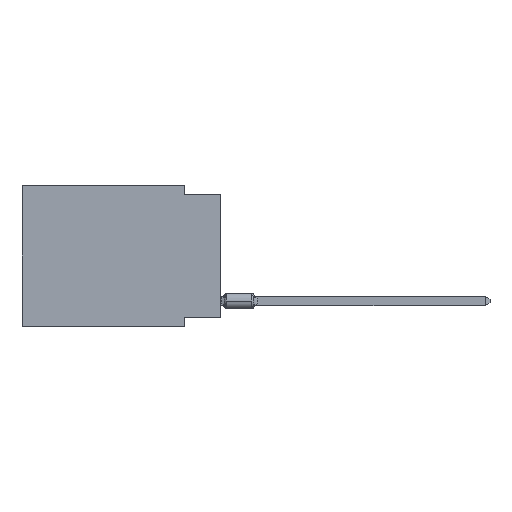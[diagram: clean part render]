
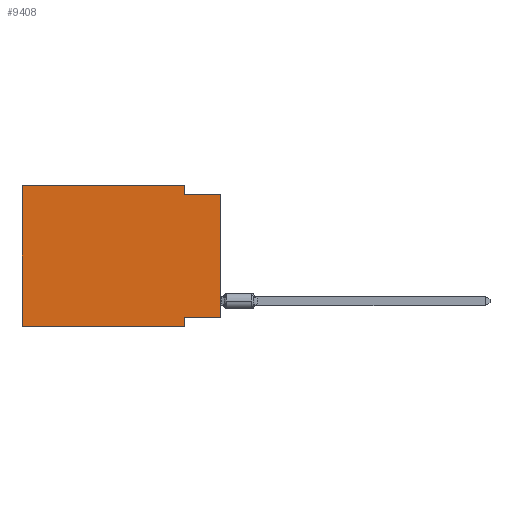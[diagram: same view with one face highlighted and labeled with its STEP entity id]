
A CAD part, left-side view. The second image highlights one B-rep face of the part: STEP entity #9408.
In plain terms, the highlighted planar face has unit normal (-1, 0, 0).
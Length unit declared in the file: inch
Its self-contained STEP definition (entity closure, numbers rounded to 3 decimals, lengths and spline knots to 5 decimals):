
#758 = VERTEX_POINT ( 'NONE', #49274 ) ;
#1329 = VERTEX_POINT ( 'NONE', #6294 ) ;
#2102 = LINE ( 'NONE', #21985, #46123 ) ;
#3447 = VERTEX_POINT ( 'NONE', #30160 ) ;
#4110 = EDGE_CURVE ( 'NONE', #7609, #20637, #10798, .T. ) ;
#5303 = EDGE_CURVE ( 'NONE', #758, #7689, #37241, .T. ) ;
#6239 = ORIENTED_EDGE ( 'NONE', *, *, #4110, .F. ) ;
#6294 = CARTESIAN_POINT ( 'NONE',  ( 0., 0.1, -0.39 ) ) ;
#6983 = LINE ( 'NONE', #15565, #15666 ) ;
#7049 = AXIS2_PLACEMENT_3D ( 'NONE', #50666, #11181, #33478 ) ;
#7492 = ORIENTED_EDGE ( 'NONE', *, *, #36009, .F. ) ;
#7609 = VERTEX_POINT ( 'NONE', #50224 ) ;
#7689 = VERTEX_POINT ( 'NONE', #36211 ) ;
#7884 = VECTOR ( 'NONE', #9864, 39.37008 ) ;
#9135 = VECTOR ( 'NONE', #55776, 39.37008 ) ;
#9408 = ADVANCED_FACE ( 'NONE', ( #32930 ), #41786, .F. ) ;
#9797 = VERTEX_POINT ( 'NONE', #33981 ) ;
#9864 = DIRECTION ( 'NONE',  ( 0., -1., 0. ) ) ;
#10026 = VECTOR ( 'NONE', #50419, 39.37008 ) ;
#10798 = LINE ( 'NONE', #19971, #32415 ) ;
#11181 = DIRECTION ( 'NONE',  ( 1., 0., 0. ) ) ;
#13975 = DIRECTION ( 'NONE',  ( 0., 0., 1. ) ) ;
#14082 = CARTESIAN_POINT ( 'NONE',  ( 0., 0.55, -0.39 ) ) ;
#14821 = CARTESIAN_POINT ( 'NONE',  ( 0., 0., 0. ) ) ;
#15501 = CARTESIAN_POINT ( 'NONE',  ( 0., 0., -0.365 ) ) ;
#15565 = CARTESIAN_POINT ( 'NONE',  ( 0., 0.1, -0.39 ) ) ;
#15666 = VECTOR ( 'NONE', #24439, 39.37008 ) ;
#15676 = DIRECTION ( 'NONE',  ( 0., 0., -1. ) ) ;
#17599 = EDGE_CURVE ( 'NONE', #38667, #1329, #40134, .T. ) ;
#18742 = ORIENTED_EDGE ( 'NONE', *, *, #40873, .F. ) ;
#19304 = VECTOR ( 'NONE', #13975, 39.37008 ) ;
#19971 = CARTESIAN_POINT ( 'NONE',  ( 0., 0.1, 0. ) ) ;
#20637 = VERTEX_POINT ( 'NONE', #37688 ) ;
#21985 = CARTESIAN_POINT ( 'NONE',  ( 0., 0.55, 0. ) ) ;
#24439 = DIRECTION ( 'NONE',  ( 0., 0., -1. ) ) ;
#24874 = CARTESIAN_POINT ( 'NONE',  ( 0., 0.55, 0. ) ) ;
#26428 = EDGE_CURVE ( 'NONE', #758, #3447, #53451, .T. ) ;
#30160 = CARTESIAN_POINT ( 'NONE',  ( 0., 0., -0.025 ) ) ;
#31531 = DIRECTION ( 'NONE',  ( 0., -1., 0. ) ) ;
#32415 = VECTOR ( 'NONE', #15676, 39.37008 ) ;
#32729 = DIRECTION ( 'NONE',  ( 0., -1., 0. ) ) ;
#32930 = FACE_OUTER_BOUND ( 'NONE', #48651, .T. ) ;
#33478 = DIRECTION ( 'NONE',  ( 0., 0., -1. ) ) ;
#33981 = CARTESIAN_POINT ( 'NONE',  ( 0., 0.55, 0. ) ) ;
#34879 = ORIENTED_EDGE ( 'NONE', *, *, #26428, .T. ) ;
#36009 = EDGE_CURVE ( 'NONE', #38667, #9797, #47151, .T. ) ;
#36187 = LINE ( 'NONE', #48504, #7884 ) ;
#36211 = CARTESIAN_POINT ( 'NONE',  ( 0., 0.1, -0.365 ) ) ;
#37241 = LINE ( 'NONE', #15501, #10026 ) ;
#37487 = VECTOR ( 'NONE', #31531, 39.37008 ) ;
#37688 = CARTESIAN_POINT ( 'NONE',  ( 0., 0.1, -0.025 ) ) ;
#38667 = VERTEX_POINT ( 'NONE', #40087 ) ;
#40087 = CARTESIAN_POINT ( 'NONE',  ( 0., 0.55, -0.39 ) ) ;
#40134 = LINE ( 'NONE', #14082, #37487 ) ;
#40413 = ORIENTED_EDGE ( 'NONE', *, *, #5303, .F. ) ;
#40873 = EDGE_CURVE ( 'NONE', #7689, #1329, #6983, .T. ) ;
#41786 = PLANE ( 'NONE',  #7049 ) ;
#44059 = ORIENTED_EDGE ( 'NONE', *, *, #17599, .T. ) ;
#44582 = ORIENTED_EDGE ( 'NONE', *, *, #45835, .F. ) ;
#45835 = EDGE_CURVE ( 'NONE', #9797, #7609, #2102, .T. ) ;
#46123 = VECTOR ( 'NONE', #32729, 39.37008 ) ;
#47151 = LINE ( 'NONE', #24874, #9135 ) ;
#48504 = CARTESIAN_POINT ( 'NONE',  ( 0., 0., -0.025 ) ) ;
#48651 = EDGE_LOOP ( 'NONE', ( #34879, #54996, #6239, #44582, #7492, #44059, #18742, #40413 ) ) ;
#49274 = CARTESIAN_POINT ( 'NONE',  ( 0., 0., -0.365 ) ) ;
#50224 = CARTESIAN_POINT ( 'NONE',  ( 0., 0.1, 0. ) ) ;
#50419 = DIRECTION ( 'NONE',  ( 0., 1., 0. ) ) ;
#50666 = CARTESIAN_POINT ( 'NONE',  ( 0., 0.55, 0. ) ) ;
#53451 = LINE ( 'NONE', #14821, #19304 ) ;
#53713 = EDGE_CURVE ( 'NONE', #20637, #3447, #36187, .T. ) ;
#54996 = ORIENTED_EDGE ( 'NONE', *, *, #53713, .F. ) ;
#55776 = DIRECTION ( 'NONE',  ( 0., 0., 1. ) ) ;
